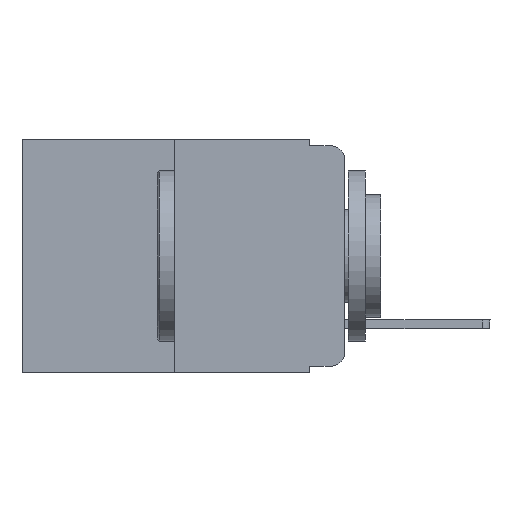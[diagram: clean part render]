
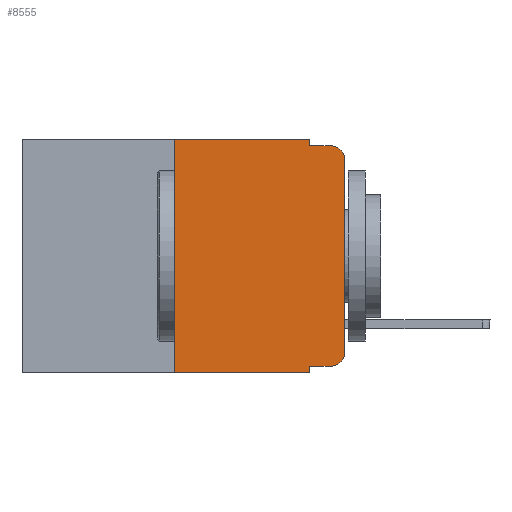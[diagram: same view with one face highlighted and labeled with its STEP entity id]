
A CAD part, left-side view. The second image highlights one B-rep face of the part: STEP entity #8555.
In plain terms, the highlighted planar face has unit normal (-1, 0, 0).
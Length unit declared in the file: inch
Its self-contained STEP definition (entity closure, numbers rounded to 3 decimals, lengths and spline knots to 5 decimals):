
#59 = DIRECTION ( 'NONE',  ( 0., -1., 0. ) ) ;
#342 = VERTEX_POINT ( 'NONE', #5364 ) ;
#405 = CARTESIAN_POINT ( 'NONE',  ( 0., 0.02, -0.01 ) ) ;
#454 = LINE ( 'NONE', #18771, #3454 ) ;
#764 = VERTEX_POINT ( 'NONE', #18480 ) ;
#1484 = VERTEX_POINT ( 'NONE', #24106 ) ;
#1506 = ORIENTED_EDGE ( 'NONE', *, *, #22165, .F. ) ;
#1760 = CARTESIAN_POINT ( 'NONE',  ( 0., 0.051, -0.343 ) ) ;
#1812 = CARTESIAN_POINT ( 'NONE',  ( 0., 0.051, -0.01 ) ) ;
#1893 = EDGE_CURVE ( 'NONE', #8345, #9198, #4903, .T. ) ;
#1985 = LINE ( 'NONE', #17679, #11247 ) ;
#2412 = VECTOR ( 'NONE', #59, 39.37008 ) ;
#2845 = ORIENTED_EDGE ( 'NONE', *, *, #1893, .F. ) ;
#2948 = VERTEX_POINT ( 'NONE', #7166 ) ;
#3454 = VECTOR ( 'NONE', #14940, 39.37008 ) ;
#4157 = EDGE_CURVE ( 'NONE', #1484, #764, #4525, .T. ) ;
#4377 = AXIS2_PLACEMENT_3D ( 'NONE', #12424, #18044, #18203 ) ;
#4525 = LINE ( 'NONE', #5033, #15497 ) ;
#4661 = EDGE_CURVE ( 'NONE', #764, #12199, #12525, .T. ) ;
#4787 = EDGE_LOOP ( 'NONE', ( #13242, #8293, #15680, #1506, #10786, #2845, #7622, #22350, #4792, #16923 ) ) ;
#4792 = ORIENTED_EDGE ( 'NONE', *, *, #17401, .T. ) ;
#4903 = LINE ( 'NONE', #16476, #22680 ) ;
#4971 = DIRECTION ( 'NONE',  ( 0., -1., 0. ) ) ;
#5033 = CARTESIAN_POINT ( 'NONE',  ( 0., 0., 0. ) ) ;
#5039 = DIRECTION ( 'NONE',  ( 1., 0., 0. ) ) ;
#5364 = CARTESIAN_POINT ( 'NONE',  ( 0., 0.051, 0. ) ) ;
#5636 = CARTESIAN_POINT ( 'NONE',  ( 0., 0.02, -0.333 ) ) ;
#6045 = VECTOR ( 'NONE', #16548, 39.37008 ) ;
#6536 = VERTEX_POINT ( 'NONE', #1812 ) ;
#6608 = DIRECTION ( 'NONE',  ( 0., -1., 0. ) ) ;
#6692 = DIRECTION ( 'NONE',  ( 0., 0., -1. ) ) ;
#6843 = PLANE ( 'NONE',  #15891 ) ;
#6918 = DIRECTION ( 'NONE',  ( 0., 0., 1. ) ) ;
#7166 = CARTESIAN_POINT ( 'NONE',  ( 0., 0.051, -0.333 ) ) ;
#7622 = ORIENTED_EDGE ( 'NONE', *, *, #21344, .T. ) ;
#8221 = VECTOR ( 'NONE', #4971, 39.37008 ) ;
#8293 = ORIENTED_EDGE ( 'NONE', *, *, #4661, .T. ) ;
#8345 = VERTEX_POINT ( 'NONE', #15787 ) ;
#8555 = ADVANCED_FACE ( 'NONE', ( #19998 ), #6843, .F. ) ;
#8627 = CARTESIAN_POINT ( 'NONE',  ( 0., 0.051, 0. ) ) ;
#9198 = VERTEX_POINT ( 'NONE', #19935 ) ;
#10786 = ORIENTED_EDGE ( 'NONE', *, *, #14913, .F. ) ;
#11151 = DIRECTION ( 'NONE',  ( 0., 0., -1. ) ) ;
#11247 = VECTOR ( 'NONE', #6608, 39.37008 ) ;
#11492 = CARTESIAN_POINT ( 'NONE',  ( 0., 0.473, 0. ) ) ;
#12143 = VERTEX_POINT ( 'NONE', #5636 ) ;
#12199 = VERTEX_POINT ( 'NONE', #405 ) ;
#12248 = CARTESIAN_POINT ( 'NONE',  ( 0., 0.473, -0.343 ) ) ;
#12424 = CARTESIAN_POINT ( 'NONE',  ( 0., 0.02, -0.03 ) ) ;
#12525 = CIRCLE ( 'NONE', #4377, 0.02 ) ;
#13242 = ORIENTED_EDGE ( 'NONE', *, *, #4157, .T. ) ;
#14585 = LINE ( 'NONE', #11492, #2412 ) ;
#14780 = DIRECTION ( 'NONE',  ( -1., 0., 0. ) ) ;
#14913 = EDGE_CURVE ( 'NONE', #9198, #342, #14585, .T. ) ;
#14940 = DIRECTION ( 'NONE',  ( 0., 0., -1. ) ) ;
#15497 = VECTOR ( 'NONE', #6918, 39.37008 ) ;
#15680 = ORIENTED_EDGE ( 'NONE', *, *, #21377, .F. ) ;
#15787 = CARTESIAN_POINT ( 'NONE',  ( 0., 0.25, -0.343 ) ) ;
#15839 = DIRECTION ( 'NONE',  ( 0., -1., 0. ) ) ;
#15853 = VERTEX_POINT ( 'NONE', #1760 ) ;
#15891 = AXIS2_PLACEMENT_3D ( 'NONE', #16396, #5039, #6692 ) ;
#16224 = DIRECTION ( 'NONE',  ( 0., 0., 1. ) ) ;
#16396 = CARTESIAN_POINT ( 'NONE',  ( 0., 0.473, 0. ) ) ;
#16476 = CARTESIAN_POINT ( 'NONE',  ( 0., 0.25, 0. ) ) ;
#16497 = AXIS2_PLACEMENT_3D ( 'NONE', #22227, #14780, #11151 ) ;
#16548 = DIRECTION ( 'NONE',  ( 0., 0., -1. ) ) ;
#16807 = LINE ( 'NONE', #23526, #8221 ) ;
#16923 = ORIENTED_EDGE ( 'NONE', *, *, #17101, .T. ) ;
#17101 = EDGE_CURVE ( 'NONE', #12143, #1484, #23369, .T. ) ;
#17348 = LINE ( 'NONE', #8627, #6045 ) ;
#17401 = EDGE_CURVE ( 'NONE', #2948, #12143, #1985, .T. ) ;
#17679 = CARTESIAN_POINT ( 'NONE',  ( 0., 0.051, -0.333 ) ) ;
#17715 = LINE ( 'NONE', #12248, #18300 ) ;
#18044 = DIRECTION ( 'NONE',  ( -1., 0., 0. ) ) ;
#18203 = DIRECTION ( 'NONE',  ( 0., 0., -1. ) ) ;
#18300 = VECTOR ( 'NONE', #15839, 39.37008 ) ;
#18480 = CARTESIAN_POINT ( 'NONE',  ( 0., 0., -0.03 ) ) ;
#18771 = CARTESIAN_POINT ( 'NONE',  ( 0., 0.051, 0. ) ) ;
#19935 = CARTESIAN_POINT ( 'NONE',  ( 0., 0.25, 0. ) ) ;
#19998 = FACE_OUTER_BOUND ( 'NONE', #4787, .T. ) ;
#21176 = EDGE_CURVE ( 'NONE', #2948, #15853, #454, .T. ) ;
#21344 = EDGE_CURVE ( 'NONE', #8345, #15853, #17715, .T. ) ;
#21377 = EDGE_CURVE ( 'NONE', #6536, #12199, #16807, .T. ) ;
#22165 = EDGE_CURVE ( 'NONE', #342, #6536, #17348, .T. ) ;
#22227 = CARTESIAN_POINT ( 'NONE',  ( 0., 0.02, -0.313 ) ) ;
#22350 = ORIENTED_EDGE ( 'NONE', *, *, #21176, .F. ) ;
#22680 = VECTOR ( 'NONE', #16224, 39.37008 ) ;
#23369 = CIRCLE ( 'NONE', #16497, 0.02 ) ;
#23526 = CARTESIAN_POINT ( 'NONE',  ( 0., 0.051, -0.01 ) ) ;
#24106 = CARTESIAN_POINT ( 'NONE',  ( 0., 0., -0.313 ) ) ;
